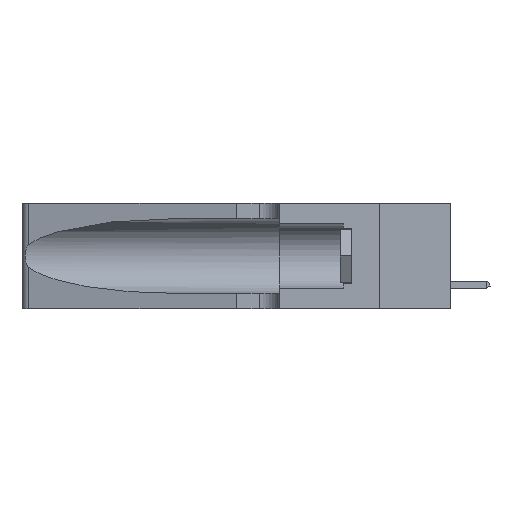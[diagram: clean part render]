
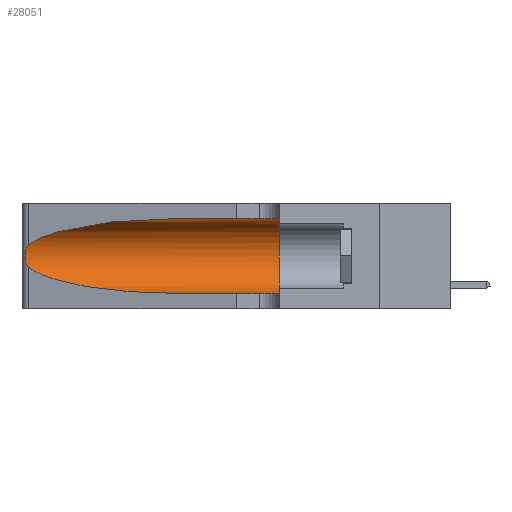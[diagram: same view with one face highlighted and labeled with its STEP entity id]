
A CAD part, left-side view. The second image highlights one B-rep face of the part: STEP entity #28051.
In plain terms, the highlighted cylindrical face has radius 3.308 mm (diameter 6.617 mm), a partial arc.
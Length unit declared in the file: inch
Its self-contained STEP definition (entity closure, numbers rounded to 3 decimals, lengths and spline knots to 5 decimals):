
#58 = CARTESIAN_POINT ( 'NONE',  ( 0.2373, 1.15595, 0.28018 ) ) ;
#81 = ORIENTED_EDGE ( 'NONE', *, *, #35596, .F. ) ;
#179 = CARTESIAN_POINT ( 'NONE',  ( 0.1305, 0.72297, 0.31525 ) ) ;
#451 = CARTESIAN_POINT ( 'NONE',  ( 0.25487, 1.22718, 0.22369 ) ) ;
#864 = EDGE_CURVE ( 'NONE', #2738, #38036, #4217, .T. ) ;
#1051 = CYLINDRICAL_SURFACE ( 'NONE', #26130, 0.13025 ) ;
#1678 = CARTESIAN_POINT ( 'NONE',  ( 0.1305, 0.72297, 0.31525 ) ) ;
#2738 = VERTEX_POINT ( 'NONE', #1678 ) ;
#3013 = CARTESIAN_POINT ( 'NONE',  ( 0.1305, 0.35, 0.185 ) ) ;
#4217 =( BOUNDED_CURVE ( )  B_SPLINE_CURVE ( 3, ( #179, #21412, #58, #451 ),
 .UNSPECIFIED., .F., .F. ) 
 B_SPLINE_CURVE_WITH_KNOTS ( ( 4, 4 ),
 ( 1.5708, 2.84003 ),
 .UNSPECIFIED. ) 
 CURVE ( )  GEOMETRIC_REPRESENTATION_ITEM ( )  RATIONAL_B_SPLINE_CURVE ( ( 1., 0.87, 0.87, 1. ) ) 
 REPRESENTATION_ITEM ( '' )  );
#5440 = CARTESIAN_POINT ( 'NONE',  ( 0.25789, 1.23486, 0.15765 ) ) ;
#6597 = DIRECTION ( 'NONE',  ( 0., 1., 0. ) ) ;
#7205 = CARTESIAN_POINT ( 'NONE',  ( 0.1305, 0.72297, 0.05475 ) ) ;
#8059 = CARTESIAN_POINT ( 'NONE',  ( 0.25854, 1.2359, 0.20912 ) ) ;
#8760 = DIRECTION ( 'NONE',  ( 0., -1., 0. ) ) ;
#8842 = CARTESIAN_POINT ( 'NONE',  ( 0.26017, 1.23833, 0.17102 ) ) ;
#9157 = CARTESIAN_POINT ( 'NONE',  ( 0.25487, 1.22718, 0.14631 ) ) ;
#11150 = VECTOR ( 'NONE', #8760, 39.37008 ) ;
#11731 = CARTESIAN_POINT ( 'NONE',  ( 0.25639, 1.23184, 0.21858 ) ) ;
#12755 = EDGE_CURVE ( 'NONE', #2738, #40957, #44319, .T. ) ;
#13361 = VERTEX_POINT ( 'NONE', #40798 ) ;
#15167 = VECTOR ( 'NONE', #26818, 39.37008 ) ;
#20057 =( BOUNDED_CURVE ( )  B_SPLINE_CURVE ( 3, ( #23004, #29600, #33441, #44003 ),
 .UNSPECIFIED., .F., .F. ) 
 B_SPLINE_CURVE_WITH_KNOTS ( ( 4, 4 ),
 ( 3.44316, 4.71239 ),
 .UNSPECIFIED. ) 
 CURVE ( )  GEOMETRIC_REPRESENTATION_ITEM ( )  RATIONAL_B_SPLINE_CURVE ( ( 1., 0.87, 0.87, 1. ) ) 
 REPRESENTATION_ITEM ( '' )  );
#20671 = ORIENTED_EDGE ( 'NONE', *, *, #41815, .T. ) ;
#21289 = CARTESIAN_POINT ( 'NONE',  ( 0.25487, 1.22718, 0.22369 ) ) ;
#21412 = CARTESIAN_POINT ( 'NONE',  ( 0.18966, 0.96281, 0.31525 ) ) ;
#21583 = CARTESIAN_POINT ( 'NONE',  ( 0.25787, 1.23484, 0.2124 ) ) ;
#22062 = CARTESIAN_POINT ( 'NONE',  ( 0.26018, 1.23835, 0.19895 ) ) ;
#23004 = CARTESIAN_POINT ( 'NONE',  ( 0.25487, 1.22718, 0.14631 ) ) ;
#23600 = CARTESIAN_POINT ( 'NONE',  ( 0.1305, 1.61858, 0.31525 ) ) ;
#24363 = ORIENTED_EDGE ( 'NONE', *, *, #864, .T. ) ;
#25147 = ORIENTED_EDGE ( 'NONE', *, *, #27075, .T. ) ;
#26130 = AXIS2_PLACEMENT_3D ( 'NONE', #34434, #38245, #38823 ) ;
#26818 = DIRECTION ( 'NONE',  ( 0., -1., 0. ) ) ;
#27002 = CARTESIAN_POINT ( 'NONE',  ( 0.25487, 1.22718, 0.14631 ) ) ;
#27021 = EDGE_CURVE ( 'NONE', #29839, #13361, #27210, .T. ) ;
#27075 = EDGE_CURVE ( 'NONE', #38036, #41835, #28226, .T. ) ;
#27210 = LINE ( 'NONE', #40551, #11150 ) ;
#28051 = ADVANCED_FACE ( 'NONE', ( #37402 ), #1051, .F. ) ;
#28226 = B_SPLINE_CURVE_WITH_KNOTS ( 'NONE', 3,
 ( #39546, #42922, #11731, #21583, #8059, #22062, #40177, #43377, #8842, #36956, #5440, #37115, #34349, #27002 ),
 .UNSPECIFIED., .F., .F.,
 ( 4, 2, 2, 2, 2, 2, 4 ),
 ( 0., 0.00027, 0.00053, 0.00107, 0.0016, 0.00187, 0.00214 ),
 .UNSPECIFIED. ) ;
#29600 = CARTESIAN_POINT ( 'NONE',  ( 0.2373, 1.15595, 0.08982 ) ) ;
#29839 = VERTEX_POINT ( 'NONE', #7205 ) ;
#30340 = ORIENTED_EDGE ( 'NONE', *, *, #12755, .F. ) ;
#33441 = CARTESIAN_POINT ( 'NONE',  ( 0.18966, 0.96281, 0.05475 ) ) ;
#33505 = ORIENTED_EDGE ( 'NONE', *, *, #27021, .T. ) ;
#34349 = CARTESIAN_POINT ( 'NONE',  ( 0.25555, 1.22993, 0.14849 ) ) ;
#34434 = CARTESIAN_POINT ( 'NONE',  ( 0.1305, 1.61858, 0.185 ) ) ;
#35596 = EDGE_CURVE ( 'NONE', #40957, #13361, #39380, .T. ) ;
#36956 = CARTESIAN_POINT ( 'NONE',  ( 0.25856, 1.23593, 0.16098 ) ) ;
#37115 = CARTESIAN_POINT ( 'NONE',  ( 0.25639, 1.23186, 0.15144 ) ) ;
#37402 = FACE_OUTER_BOUND ( 'NONE', #44823, .T. ) ;
#37646 = DIRECTION ( 'NONE',  ( 0., 0., 1. ) ) ;
#38036 = VERTEX_POINT ( 'NONE', #21289 ) ;
#38245 = DIRECTION ( 'NONE',  ( 0., -1., 0. ) ) ;
#38823 = DIRECTION ( 'NONE',  ( 0., 0., -1. ) ) ;
#39380 = CIRCLE ( 'NONE', #40457, 0.13025 ) ;
#39546 = CARTESIAN_POINT ( 'NONE',  ( 0.25487, 1.22718, 0.22369 ) ) ;
#40177 = CARTESIAN_POINT ( 'NONE',  ( 0.26075, 1.23896, 0.19203 ) ) ;
#40457 = AXIS2_PLACEMENT_3D ( 'NONE', #3013, #6597, #37646 ) ;
#40551 = CARTESIAN_POINT ( 'NONE',  ( 0.1305, 1.61858, 0.05475 ) ) ;
#40798 = CARTESIAN_POINT ( 'NONE',  ( 0.1305, 0.35, 0.05475 ) ) ;
#40957 = VERTEX_POINT ( 'NONE', #43127 ) ;
#41815 = EDGE_CURVE ( 'NONE', #41835, #29839, #20057, .T. ) ;
#41835 = VERTEX_POINT ( 'NONE', #9157 ) ;
#42922 = CARTESIAN_POINT ( 'NONE',  ( 0.25555, 1.22994, 0.2215 ) ) ;
#43127 = CARTESIAN_POINT ( 'NONE',  ( 0.1305, 0.35, 0.31525 ) ) ;
#43377 = CARTESIAN_POINT ( 'NONE',  ( 0.26075, 1.23896, 0.178 ) ) ;
#44003 = CARTESIAN_POINT ( 'NONE',  ( 0.1305, 0.72297, 0.05475 ) ) ;
#44319 = LINE ( 'NONE', #23600, #15167 ) ;
#44823 = EDGE_LOOP ( 'NONE', ( #24363, #25147, #20671, #33505, #81, #30340 ) ) ;
